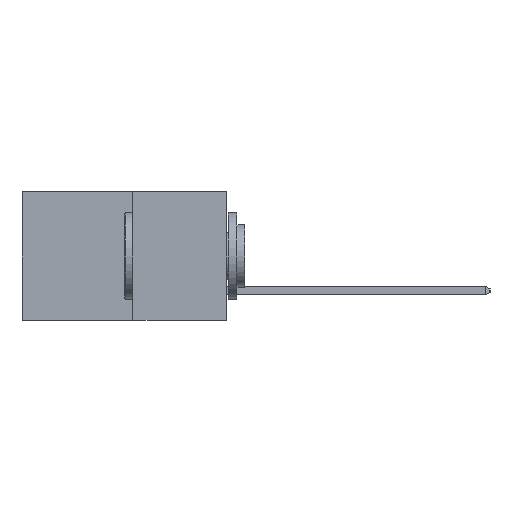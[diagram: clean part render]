
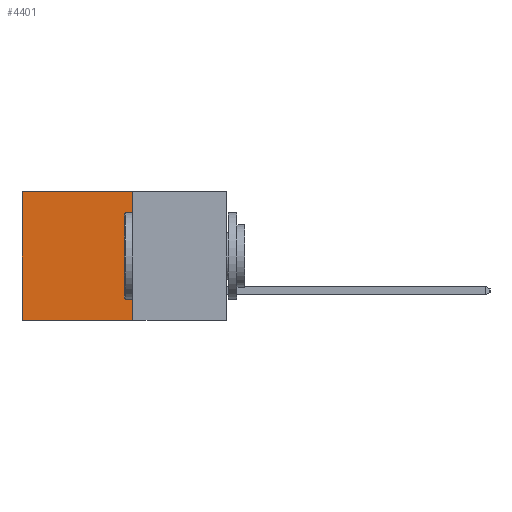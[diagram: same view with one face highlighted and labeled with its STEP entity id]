
A CAD part, left-side view. The second image highlights one B-rep face of the part: STEP entity #4401.
In plain terms, the highlighted planar face has unit normal (-1, 0, 0).
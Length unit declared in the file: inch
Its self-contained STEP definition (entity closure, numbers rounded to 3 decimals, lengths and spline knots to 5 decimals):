
#1192 = ORIENTED_EDGE ( 'NONE', *, *, #25486, .F. ) ;
#1465 = AXIS2_PLACEMENT_3D ( 'NONE', #21371, #21345, #21231 ) ;
#1762 = CARTESIAN_POINT ( 'NONE',  ( 0.277, 0.59, -0.37 ) ) ;
#1790 = VERTEX_POINT ( 'NONE', #20259 ) ;
#2185 = FACE_OUTER_BOUND ( 'NONE', #7808, .T. ) ;
#2453 = ORIENTED_EDGE ( 'NONE', *, *, #6471, .T. ) ;
#4401 = ADVANCED_FACE ( 'NONE', ( #2185 ), #18993, .F. ) ;
#4983 = VECTOR ( 'NONE', #26227, 39.37008 ) ;
#6471 = EDGE_CURVE ( 'NONE', #1790, #23563, #22398, .T. ) ;
#6639 = CARTESIAN_POINT ( 'NONE',  ( 0.277, 0.27, -0.37 ) ) ;
#7804 = VECTOR ( 'NONE', #17512, 39.37008 ) ;
#7808 = EDGE_LOOP ( 'NONE', ( #2453, #8688, #1192, #23748 ) ) ;
#8688 = ORIENTED_EDGE ( 'NONE', *, *, #16645, .F. ) ;
#8775 = DIRECTION ( 'NONE',  ( 0., 0., -1. ) ) ;
#11519 = CARTESIAN_POINT ( 'NONE',  ( 0.277, 0.27, -0.37 ) ) ;
#11943 = CARTESIAN_POINT ( 'NONE',  ( 0.277, 0.27, 0. ) ) ;
#13285 = LINE ( 'NONE', #15463, #7804 ) ;
#15463 = CARTESIAN_POINT ( 'NONE',  ( 0.277, 0.27, -0.37 ) ) ;
#16303 = VECTOR ( 'NONE', #18299, 39.37008 ) ;
#16645 = EDGE_CURVE ( 'NONE', #18120, #23563, #13285, .T. ) ;
#17512 = DIRECTION ( 'NONE',  ( 0., 1., 0. ) ) ;
#18120 = VERTEX_POINT ( 'NONE', #11519 ) ;
#18299 = DIRECTION ( 'NONE',  ( 0., 0., -1. ) ) ;
#18727 = VECTOR ( 'NONE', #8775, 39.37008 ) ;
#18993 = PLANE ( 'NONE',  #1465 ) ;
#19954 = EDGE_CURVE ( 'NONE', #26410, #1790, #26217, .T. ) ;
#20259 = CARTESIAN_POINT ( 'NONE',  ( 0.277, 0.59, 0. ) ) ;
#21231 = DIRECTION ( 'NONE',  ( 0., 0., -1. ) ) ;
#21345 = DIRECTION ( 'NONE',  ( 1., 0., 0. ) ) ;
#21371 = CARTESIAN_POINT ( 'NONE',  ( 0.277, 0.27, -0.37 ) ) ;
#22398 = LINE ( 'NONE', #1762, #16303 ) ;
#23548 = LINE ( 'NONE', #6639, #18727 ) ;
#23563 = VERTEX_POINT ( 'NONE', #26534 ) ;
#23748 = ORIENTED_EDGE ( 'NONE', *, *, #19954, .T. ) ;
#24104 = CARTESIAN_POINT ( 'NONE',  ( 0.277, 0.27, 0. ) ) ;
#25486 = EDGE_CURVE ( 'NONE', #26410, #18120, #23548, .T. ) ;
#26217 = LINE ( 'NONE', #11943, #4983 ) ;
#26227 = DIRECTION ( 'NONE',  ( 0., 1., 0. ) ) ;
#26410 = VERTEX_POINT ( 'NONE', #24104 ) ;
#26534 = CARTESIAN_POINT ( 'NONE',  ( 0.277, 0.59, -0.37 ) ) ;
